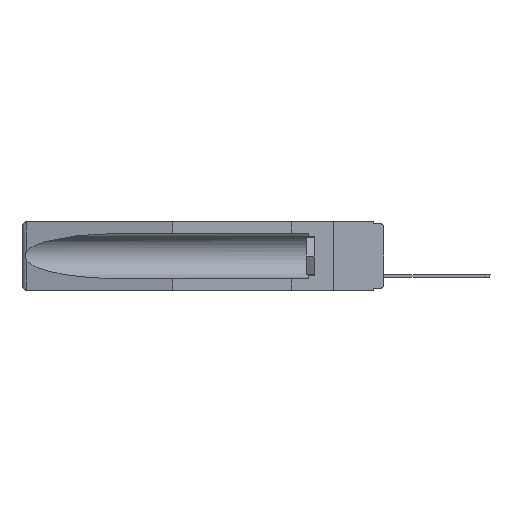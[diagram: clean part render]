
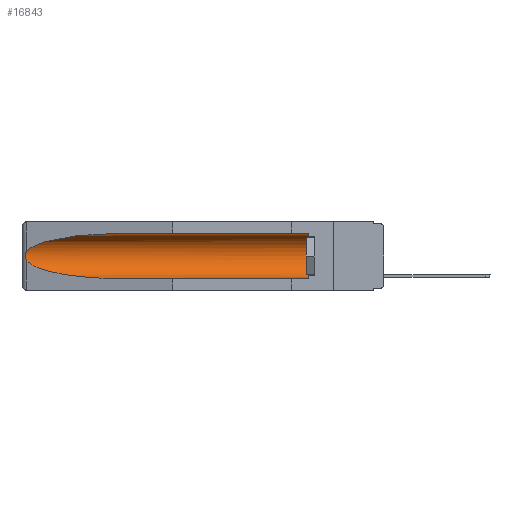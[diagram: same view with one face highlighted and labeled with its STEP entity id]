
A CAD part, left-side view. The second image highlights one B-rep face of the part: STEP entity #16843.
In plain terms, the highlighted cylindrical face has radius 2.857 mm (diameter 5.715 mm), a partial arc.
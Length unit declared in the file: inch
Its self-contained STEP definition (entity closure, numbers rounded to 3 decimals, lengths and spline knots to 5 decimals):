
#217 = LINE ( 'NONE', #1592, #12256 ) ;
#228 = DIRECTION ( 'NONE',  ( 0., 0., 1. ) ) ;
#380 = EDGE_CURVE ( 'NONE', #3847, #12876, #11211, .T. ) ;
#405 = VERTEX_POINT ( 'NONE', #8732 ) ;
#441 = ORIENTED_EDGE ( 'NONE', *, *, #14757, .F. ) ;
#659 = LINE ( 'NONE', #17187, #4853 ) ;
#900 = EDGE_CURVE ( 'NONE', #10739, #12468, #1307, .T. ) ;
#1042 = ORIENTED_EDGE ( 'NONE', *, *, #900, .T. ) ;
#1307 =( BOUNDED_CURVE ( )  B_SPLINE_CURVE ( 3, ( #19148, #16220, #2804, #8801 ),
 .UNSPECIFIED., .F., .F. ) 
 B_SPLINE_CURVE_WITH_KNOTS ( ( 4, 4 ),
 ( 0.1948, 1.5708 ),
 .UNSPECIFIED. ) 
 CURVE ( )  GEOMETRIC_REPRESENTATION_ITEM ( )  RATIONAL_B_SPLINE_CURVE ( ( 1., 0.848, 0.848, 1. ) ) 
 REPRESENTATION_ITEM ( '' )  );
#1592 = CARTESIAN_POINT ( 'NONE',  ( 0.155, -0.30754, -0.059 ) ) ;
#1645 = CARTESIAN_POINT ( 'NONE',  ( 0.2675, 1.53308, -0.17534 ) ) ;
#1707 = CYLINDRICAL_SURFACE ( 'NONE', #12044, 0.1125 ) ;
#2130 = EDGE_CURVE ( 'NONE', #12876, #10739, #5817, .T. ) ;
#2646 = CARTESIAN_POINT ( 'NONE',  ( 0.25451, 1.48313, -0.09465 ) ) ;
#2804 = CARTESIAN_POINT ( 'NONE',  ( 0.21114, 1.30732, -0.284 ) ) ;
#2968 = VERTEX_POINT ( 'NONE', #5614 ) ;
#3480 = ORIENTED_EDGE ( 'NONE', *, *, #380, .T. ) ;
#3847 = VERTEX_POINT ( 'NONE', #18253 ) ;
#4181 = CARTESIAN_POINT ( 'NONE',  ( 0.21114, 1.30732, -0.059 ) ) ;
#4418 = CARTESIAN_POINT ( 'NONE',  ( 0.26537, 1.52718, -0.14972 ) ) ;
#4783 = CARTESIAN_POINT ( 'NONE',  ( 0.26655, 1.53094, -0.18657 ) ) ;
#4853 = VECTOR ( 'NONE', #9584, 39.37008 ) ;
#5265 = EDGE_CURVE ( 'NONE', #2968, #3847, #217, .T. ) ;
#5614 = CARTESIAN_POINT ( 'NONE',  ( 0.155, 0.126, -0.059 ) ) ;
#5817 = B_SPLINE_CURVE_WITH_KNOTS ( 'NONE', 3,
 ( #15147, #13590, #7930, #12323, #13679, #1645, #6549, #4783, #15049, #18279 ),
 .UNSPECIFIED., .F., .F.,
 ( 4, 2, 2, 2, 4 ),
 ( 0., 0.00029, 0.00058, 0.00087, 0.00117 ),
 .UNSPECIFIED. ) ;
#6549 = CARTESIAN_POINT ( 'NONE',  ( 0.2673, 1.53269, -0.17917 ) ) ;
#7110 = ORIENTED_EDGE ( 'NONE', *, *, #2130, .T. ) ;
#7181 = ORIENTED_EDGE ( 'NONE', *, *, #9965, .T. ) ;
#7696 = CARTESIAN_POINT ( 'NONE',  ( 0.155, -0.30754, -0.1715 ) ) ;
#7854 = ORIENTED_EDGE ( 'NONE', *, *, #5265, .T. ) ;
#7930 = CARTESIAN_POINT ( 'NONE',  ( 0.26654, 1.53092, -0.15636 ) ) ;
#8189 = DIRECTION ( 'NONE',  ( 0., -1., 0. ) ) ;
#8732 = CARTESIAN_POINT ( 'NONE',  ( 0.155, 0.126, -0.284 ) ) ;
#8801 = CARTESIAN_POINT ( 'NONE',  ( 0.155, 1.07973, -0.284 ) ) ;
#9584 = DIRECTION ( 'NONE',  ( 0., 1., 0. ) ) ;
#9909 = EDGE_LOOP ( 'NONE', ( #3480, #7110, #1042, #441, #7181, #7854 ) ) ;
#9965 = EDGE_CURVE ( 'NONE', #405, #2968, #11302, .T. ) ;
#10739 = VERTEX_POINT ( 'NONE', #13900 ) ;
#11211 =( BOUNDED_CURVE ( )  B_SPLINE_CURVE ( 3, ( #11614, #4181, #2646, #4418 ),
 .UNSPECIFIED., .F., .F. ) 
 B_SPLINE_CURVE_WITH_KNOTS ( ( 4, 4 ),
 ( 4.71239, 6.08839 ),
 .UNSPECIFIED. ) 
 CURVE ( )  GEOMETRIC_REPRESENTATION_ITEM ( )  RATIONAL_B_SPLINE_CURVE ( ( 1., 0.848, 0.848, 1. ) ) 
 REPRESENTATION_ITEM ( '' )  );
#11302 = CIRCLE ( 'NONE', #17555, 0.1125 ) ;
#11614 = CARTESIAN_POINT ( 'NONE',  ( 0.155, 1.07973, -0.059 ) ) ;
#12034 = CARTESIAN_POINT ( 'NONE',  ( 0.155, 1.07973, -0.284 ) ) ;
#12044 = AXIS2_PLACEMENT_3D ( 'NONE', #7696, #13652, #228 ) ;
#12083 = DIRECTION ( 'NONE',  ( 0., 1., 0. ) ) ;
#12256 = VECTOR ( 'NONE', #12083, 39.37008 ) ;
#12323 = CARTESIAN_POINT ( 'NONE',  ( 0.2673, 1.5327, -0.16383 ) ) ;
#12468 = VERTEX_POINT ( 'NONE', #12034 ) ;
#12876 = VERTEX_POINT ( 'NONE', #16524 ) ;
#13590 = CARTESIAN_POINT ( 'NONE',  ( 0.26597, 1.52961, -0.15275 ) ) ;
#13652 = DIRECTION ( 'NONE',  ( 0., 1., 0. ) ) ;
#13679 = CARTESIAN_POINT ( 'NONE',  ( 0.2675, 1.53308, -0.16763 ) ) ;
#13900 = CARTESIAN_POINT ( 'NONE',  ( 0.26537, 1.52718, -0.19328 ) ) ;
#14757 = EDGE_CURVE ( 'NONE', #405, #12468, #659, .T. ) ;
#15049 = CARTESIAN_POINT ( 'NONE',  ( 0.26597, 1.5296, -0.19026 ) ) ;
#15114 = FACE_OUTER_BOUND ( 'NONE', #9909, .T. ) ;
#15147 = CARTESIAN_POINT ( 'NONE',  ( 0.26537, 1.52718, -0.14972 ) ) ;
#15597 = CARTESIAN_POINT ( 'NONE',  ( 0.155, 0.126, -0.1715 ) ) ;
#16220 = CARTESIAN_POINT ( 'NONE',  ( 0.25451, 1.48313, -0.24835 ) ) ;
#16524 = CARTESIAN_POINT ( 'NONE',  ( 0.26537, 1.52718, -0.14972 ) ) ;
#16843 = ADVANCED_FACE ( 'NONE', ( #15114 ), #1707, .F. ) ;
#17187 = CARTESIAN_POINT ( 'NONE',  ( 0.155, -0.30754, -0.284 ) ) ;
#17555 = AXIS2_PLACEMENT_3D ( 'NONE', #15597, #8189, #18640 ) ;
#18253 = CARTESIAN_POINT ( 'NONE',  ( 0.155, 1.07973, -0.059 ) ) ;
#18279 = CARTESIAN_POINT ( 'NONE',  ( 0.26537, 1.52718, -0.19328 ) ) ;
#18640 = DIRECTION ( 'NONE',  ( 0., 0., 1. ) ) ;
#19148 = CARTESIAN_POINT ( 'NONE',  ( 0.26537, 1.52718, -0.19328 ) ) ;
